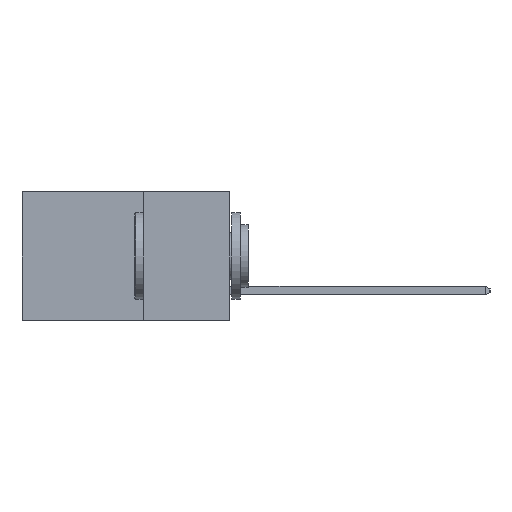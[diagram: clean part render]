
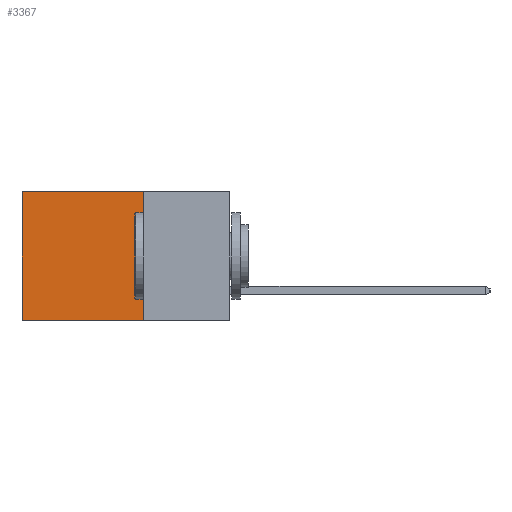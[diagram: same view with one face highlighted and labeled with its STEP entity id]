
A CAD part, left-side view. The second image highlights one B-rep face of the part: STEP entity #3367.
In plain terms, the highlighted planar face has unit normal (-1, 0, 0).
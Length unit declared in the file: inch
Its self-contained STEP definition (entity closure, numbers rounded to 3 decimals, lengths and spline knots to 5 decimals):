
#54 = CARTESIAN_POINT ( 'NONE',  ( 0.2615, 0.25, 0. ) ) ;
#117 = CARTESIAN_POINT ( 'NONE',  ( 0.2615, 0.25, -0.37 ) ) ;
#1016 = VECTOR ( 'NONE', #1844, 39.37008 ) ;
#1844 = DIRECTION ( 'NONE',  ( 0., 0., -1. ) ) ;
#2088 = ORIENTED_EDGE ( 'NONE', *, *, #7780, .T. ) ;
#2141 = CARTESIAN_POINT ( 'NONE',  ( 0.2615, 0.6, -0.37 ) ) ;
#2162 = DIRECTION ( 'NONE',  ( 0., 1., 0. ) ) ;
#2589 = DIRECTION ( 'NONE',  ( 0., 0., -1. ) ) ;
#3012 = VECTOR ( 'NONE', #2589, 39.37008 ) ;
#3342 = CARTESIAN_POINT ( 'NONE',  ( 0.2615, 0.6, 0. ) ) ;
#3367 = ADVANCED_FACE ( 'NONE', ( #4375 ), #11985, .F. ) ;
#4375 = FACE_OUTER_BOUND ( 'NONE', #15250, .T. ) ;
#4559 = CARTESIAN_POINT ( 'NONE',  ( 0.2615, 0.25, 0. ) ) ;
#4943 = DIRECTION ( 'NONE',  ( 0., 1., 0. ) ) ;
#7780 = EDGE_CURVE ( 'NONE', #17405, #7918, #13731, .T. ) ;
#7918 = VERTEX_POINT ( 'NONE', #3342 ) ;
#10058 = CARTESIAN_POINT ( 'NONE',  ( 0.2615, 0.25, -0.37 ) ) ;
#10494 = VERTEX_POINT ( 'NONE', #117 ) ;
#11985 = PLANE ( 'NONE',  #19007 ) ;
#12488 = EDGE_CURVE ( 'NONE', #7918, #16990, #13532, .T. ) ;
#12719 = CARTESIAN_POINT ( 'NONE',  ( 0.2615, 0.25, -0.37 ) ) ;
#13261 = VECTOR ( 'NONE', #4943, 39.37008 ) ;
#13532 = LINE ( 'NONE', #18786, #1016 ) ;
#13626 = LINE ( 'NONE', #10058, #17151 ) ;
#13731 = LINE ( 'NONE', #4559, #13261 ) ;
#13763 = DIRECTION ( 'NONE',  ( 0., 0., -1. ) ) ;
#13871 = DIRECTION ( 'NONE',  ( 1., 0., 0. ) ) ;
#14037 = EDGE_CURVE ( 'NONE', #17405, #10494, #15461, .T. ) ;
#14127 = ORIENTED_EDGE ( 'NONE', *, *, #19580, .F. ) ;
#15037 = CARTESIAN_POINT ( 'NONE',  ( 0.2615, 0.25, -0.37 ) ) ;
#15200 = ORIENTED_EDGE ( 'NONE', *, *, #12488, .T. ) ;
#15250 = EDGE_LOOP ( 'NONE', ( #15200, #14127, #17150, #2088 ) ) ;
#15461 = LINE ( 'NONE', #15037, #3012 ) ;
#16990 = VERTEX_POINT ( 'NONE', #2141 ) ;
#17150 = ORIENTED_EDGE ( 'NONE', *, *, #14037, .F. ) ;
#17151 = VECTOR ( 'NONE', #2162, 39.37008 ) ;
#17405 = VERTEX_POINT ( 'NONE', #54 ) ;
#18786 = CARTESIAN_POINT ( 'NONE',  ( 0.2615, 0.6, -0.37 ) ) ;
#19007 = AXIS2_PLACEMENT_3D ( 'NONE', #12719, #13871, #13763 ) ;
#19580 = EDGE_CURVE ( 'NONE', #10494, #16990, #13626, .T. ) ;
